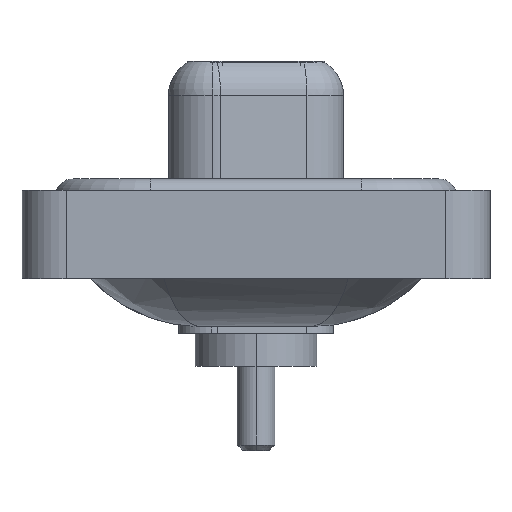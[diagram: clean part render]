
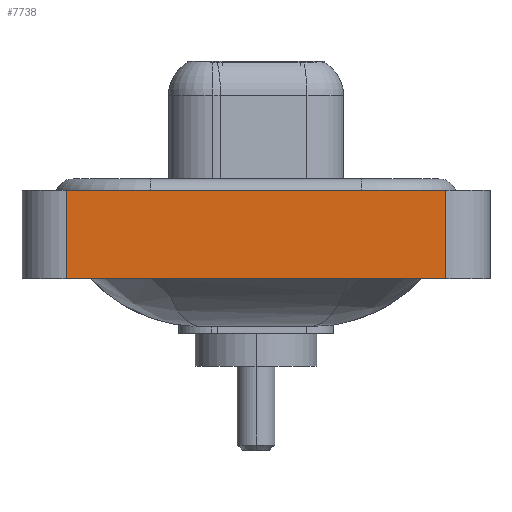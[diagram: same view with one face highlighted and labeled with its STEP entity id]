
A CAD part, left-side view. The second image highlights one B-rep face of the part: STEP entity #7738.
In plain terms, the highlighted planar face has unit normal (-1, 0, 0).
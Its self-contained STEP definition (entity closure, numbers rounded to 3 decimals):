
#87 = CARTESIAN_POINT ( 'NONE',  ( -7.25, 8.55, -3.6 ) ) ;
#632 = DIRECTION ( 'NONE',  ( 0., -1., 0. ) ) ;
#1511 = ORIENTED_EDGE ( 'NONE', *, *, #14463, .T. ) ;
#1582 = DIRECTION ( 'NONE',  ( -1., 0., 0. ) ) ;
#2062 = VERTEX_POINT ( 'NONE', #10230 ) ;
#2225 = CARTESIAN_POINT ( 'NONE',  ( -7.25, -8.55, -3.6 ) ) ;
#2865 = EDGE_CURVE ( 'NONE', #2062, #14241, #15663, .T. ) ;
#5266 = DIRECTION ( 'NONE',  ( 0., 0., 1. ) ) ;
#5740 = EDGE_CURVE ( 'NONE', #7970, #14241, #6577, .T. ) ;
#6187 = EDGE_CURVE ( 'NONE', #11991, #2062, #13662, .T. ) ;
#6345 = FACE_OUTER_BOUND ( 'NONE', #13209, .T. ) ;
#6577 = LINE ( 'NONE', #6655, #9120 ) ;
#6655 = CARTESIAN_POINT ( 'NONE',  ( -7.25, -8.55, -3.6 ) ) ;
#6752 = CARTESIAN_POINT ( 'NONE',  ( -7.25, -8.55, -3.6 ) ) ;
#7634 = DIRECTION ( 'NONE',  ( 0., 0., 1. ) ) ;
#7693 = CARTESIAN_POINT ( 'NONE',  ( -7.25, -8.55, -3.6 ) ) ;
#7738 = ADVANCED_FACE ( 'NONE', ( #6345 ), #11235, .T. ) ;
#7970 = VERTEX_POINT ( 'NONE', #2225 ) ;
#8162 = DIRECTION ( 'NONE',  ( 0., -1., 0. ) ) ;
#9120 = VECTOR ( 'NONE', #7634, 1000. ) ;
#10080 = CARTESIAN_POINT ( 'NONE',  ( -7.25, 8.55, -3.6 ) ) ;
#10163 = VECTOR ( 'NONE', #15014, 1000. ) ;
#10230 = CARTESIAN_POINT ( 'NONE',  ( -7.25, 8.55, 0.4 ) ) ;
#10732 = CARTESIAN_POINT ( 'NONE',  ( -7.25, -8.55, 0.4 ) ) ;
#10941 = VECTOR ( 'NONE', #8162, 1000. ) ;
#11235 = PLANE ( 'NONE',  #14510 ) ;
#11991 = VERTEX_POINT ( 'NONE', #87 ) ;
#12393 = CARTESIAN_POINT ( 'NONE',  ( -7.25, -8.55, 0.4 ) ) ;
#13209 = EDGE_LOOP ( 'NONE', ( #13603, #15145, #15486, #1511 ) ) ;
#13603 = ORIENTED_EDGE ( 'NONE', *, *, #5740, .T. ) ;
#13662 = LINE ( 'NONE', #10080, #10163 ) ;
#14241 = VERTEX_POINT ( 'NONE', #12393 ) ;
#14463 = EDGE_CURVE ( 'NONE', #11991, #7970, #15205, .T. ) ;
#14510 = AXIS2_PLACEMENT_3D ( 'NONE', #7693, #1582, #5266 ) ;
#15014 = DIRECTION ( 'NONE',  ( 0., 0., 1. ) ) ;
#15045 = VECTOR ( 'NONE', #632, 1000. ) ;
#15145 = ORIENTED_EDGE ( 'NONE', *, *, #2865, .F. ) ;
#15205 = LINE ( 'NONE', #6752, #15045 ) ;
#15486 = ORIENTED_EDGE ( 'NONE', *, *, #6187, .F. ) ;
#15663 = LINE ( 'NONE', #10732, #10941 ) ;
